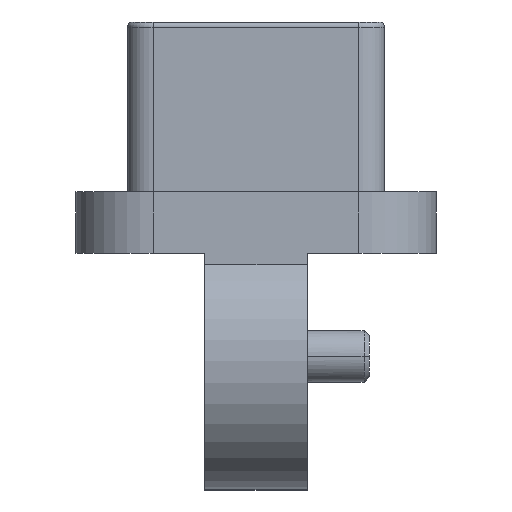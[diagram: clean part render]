
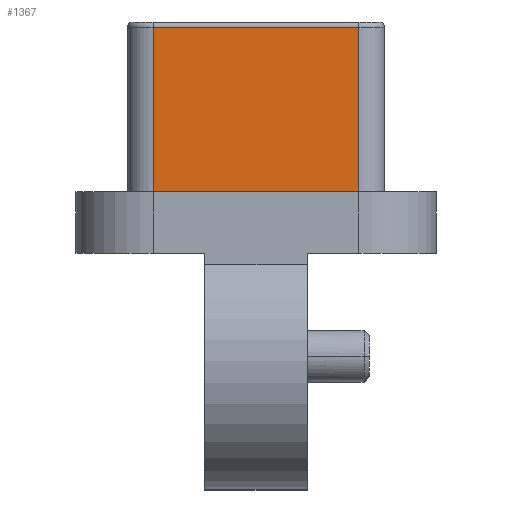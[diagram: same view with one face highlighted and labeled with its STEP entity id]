
A CAD part, left-side view. The second image highlights one B-rep face of the part: STEP entity #1367.
In plain terms, the highlighted planar face has unit normal (-1, 0, 0).
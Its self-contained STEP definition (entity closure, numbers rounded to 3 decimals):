
#644 = CARTESIAN_POINT ( 'NONE',  ( -9.65, -2., -0.1 ) ) ;
#1119 = VERTEX_POINT ( 'NONE', #5812 ) ;
#1128 = DIRECTION ( 'NONE',  ( 1., 0., 0. ) ) ;
#1213 = DIRECTION ( 'NONE',  ( 0., 0., -1. ) ) ;
#1367 = ADVANCED_FACE ( 'NONE', ( #1704 ), #4085, .F. ) ;
#1390 = CARTESIAN_POINT ( 'NONE',  ( -9.65, 2., -3.3 ) ) ;
#1704 = FACE_OUTER_BOUND ( 'NONE', #2790, .T. ) ;
#1881 = DIRECTION ( 'NONE',  ( 0., 0., 1. ) ) ;
#1908 = EDGE_CURVE ( 'NONE', #3953, #1119, #4839, .T. ) ;
#2312 = ORIENTED_EDGE ( 'NONE', *, *, #4478, .T. ) ;
#2790 = EDGE_LOOP ( 'NONE', ( #3194, #2312, #3676, #6343 ) ) ;
#2916 = VERTEX_POINT ( 'NONE', #6431 ) ;
#3032 = DIRECTION ( 'NONE',  ( 0., 1., 0. ) ) ;
#3194 = ORIENTED_EDGE ( 'NONE', *, *, #5721, .T. ) ;
#3504 = DIRECTION ( 'NONE',  ( 0., 1., 0. ) ) ;
#3518 = CARTESIAN_POINT ( 'NONE',  ( -9.65, -2., -3.3 ) ) ;
#3676 = ORIENTED_EDGE ( 'NONE', *, *, #1908, .T. ) ;
#3770 = DIRECTION ( 'NONE',  ( 0., -1., 0. ) ) ;
#3953 = VERTEX_POINT ( 'NONE', #3518 ) ;
#3987 = VECTOR ( 'NONE', #3032, 1000. ) ;
#3991 = VECTOR ( 'NONE', #1881, 1000. ) ;
#4085 = PLANE ( 'NONE',  #6727 ) ;
#4172 = LINE ( 'NONE', #6544, #7168 ) ;
#4478 = EDGE_CURVE ( 'NONE', #4840, #3953, #6721, .T. ) ;
#4839 = LINE ( 'NONE', #7217, #3991 ) ;
#4840 = VERTEX_POINT ( 'NONE', #6034 ) ;
#5721 = EDGE_CURVE ( 'NONE', #2916, #4840, #4172, .T. ) ;
#5812 = CARTESIAN_POINT ( 'NONE',  ( -9.65, -2., -0.1 ) ) ;
#5981 = LINE ( 'NONE', #644, #3987 ) ;
#6015 = VECTOR ( 'NONE', #3770, 1000. ) ;
#6034 = CARTESIAN_POINT ( 'NONE',  ( -9.65, 2., -3.3 ) ) ;
#6343 = ORIENTED_EDGE ( 'NONE', *, *, #7099, .T. ) ;
#6431 = CARTESIAN_POINT ( 'NONE',  ( -9.65, 2., -0.1 ) ) ;
#6458 = CARTESIAN_POINT ( 'NONE',  ( -9.65, 0., -1.7 ) ) ;
#6544 = CARTESIAN_POINT ( 'NONE',  ( -9.65, 2., -0.1 ) ) ;
#6721 = LINE ( 'NONE', #1390, #6015 ) ;
#6727 = AXIS2_PLACEMENT_3D ( 'NONE', #6458, #1128, #3504 ) ;
#7099 = EDGE_CURVE ( 'NONE', #1119, #2916, #5981, .T. ) ;
#7168 = VECTOR ( 'NONE', #1213, 1000. ) ;
#7217 = CARTESIAN_POINT ( 'NONE',  ( -9.65, -2., -3.3 ) ) ;
